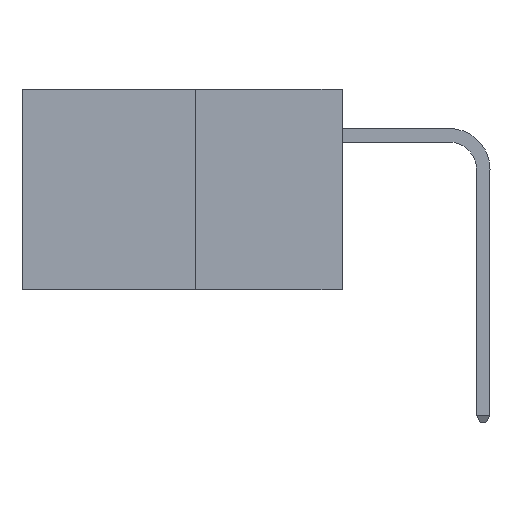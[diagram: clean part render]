
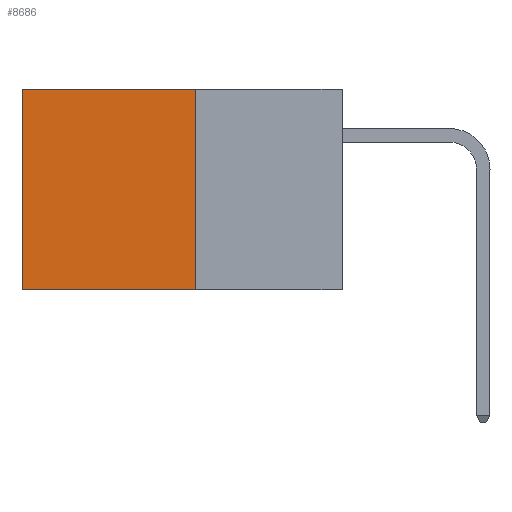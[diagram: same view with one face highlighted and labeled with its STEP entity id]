
A CAD part, left-side view. The second image highlights one B-rep face of the part: STEP entity #8686.
In plain terms, the highlighted planar face has unit normal (-1, 0, 0).
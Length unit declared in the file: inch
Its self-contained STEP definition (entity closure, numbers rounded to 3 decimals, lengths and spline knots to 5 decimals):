
#149 = LINE ( 'NONE', #12053, #574 ) ;
#518 = ORIENTED_EDGE ( 'NONE', *, *, #13031, .F. ) ;
#574 = VECTOR ( 'NONE', #11943, 39.37008 ) ;
#851 = CARTESIAN_POINT ( 'NONE',  ( 0.277, 0.27, 0. ) ) ;
#1091 = VERTEX_POINT ( 'NONE', #7757 ) ;
#2084 = VERTEX_POINT ( 'NONE', #6373 ) ;
#2275 = VERTEX_POINT ( 'NONE', #7153 ) ;
#2675 = DIRECTION ( 'NONE',  ( 1., 0., 0. ) ) ;
#2808 = LINE ( 'NONE', #12926, #16389 ) ;
#3205 = CARTESIAN_POINT ( 'NONE',  ( 0.277, 0.27, -0.37 ) ) ;
#3244 = VECTOR ( 'NONE', #12481, 39.37008 ) ;
#4827 = DIRECTION ( 'NONE',  ( 0., 1., 0. ) ) ;
#4994 = CARTESIAN_POINT ( 'NONE',  ( 0.277, 0.27, 0. ) ) ;
#5032 = EDGE_CURVE ( 'NONE', #2084, #2275, #149, .T. ) ;
#5058 = EDGE_CURVE ( 'NONE', #12966, #2084, #16876, .T. ) ;
#6373 = CARTESIAN_POINT ( 'NONE',  ( 0.277, 0.59, 0. ) ) ;
#6388 = LINE ( 'NONE', #3205, #3244 ) ;
#7064 = ORIENTED_EDGE ( 'NONE', *, *, #5058, .T. ) ;
#7153 = CARTESIAN_POINT ( 'NONE',  ( 0.277, 0.59, -0.37 ) ) ;
#7515 = ORIENTED_EDGE ( 'NONE', *, *, #13650, .F. ) ;
#7705 = DIRECTION ( 'NONE',  ( 0., 1., 0. ) ) ;
#7757 = CARTESIAN_POINT ( 'NONE',  ( 0.277, 0.27, -0.37 ) ) ;
#8004 = PLANE ( 'NONE',  #12241 ) ;
#8426 = ORIENTED_EDGE ( 'NONE', *, *, #5032, .T. ) ;
#8686 = ADVANCED_FACE ( 'NONE', ( #11304 ), #8004, .F. ) ;
#10797 = VECTOR ( 'NONE', #4827, 39.37008 ) ;
#11304 = FACE_OUTER_BOUND ( 'NONE', #13478, .T. ) ;
#11943 = DIRECTION ( 'NONE',  ( 0., 0., -1. ) ) ;
#11980 = DIRECTION ( 'NONE',  ( 0., 0., -1. ) ) ;
#12053 = CARTESIAN_POINT ( 'NONE',  ( 0.277, 0.59, -0.37 ) ) ;
#12241 = AXIS2_PLACEMENT_3D ( 'NONE', #17046, #2675, #11980 ) ;
#12481 = DIRECTION ( 'NONE',  ( 0., 0., -1. ) ) ;
#12926 = CARTESIAN_POINT ( 'NONE',  ( 0.277, 0.27, -0.37 ) ) ;
#12966 = VERTEX_POINT ( 'NONE', #851 ) ;
#13031 = EDGE_CURVE ( 'NONE', #1091, #2275, #2808, .T. ) ;
#13478 = EDGE_LOOP ( 'NONE', ( #8426, #518, #7515, #7064 ) ) ;
#13650 = EDGE_CURVE ( 'NONE', #12966, #1091, #6388, .T. ) ;
#16389 = VECTOR ( 'NONE', #7705, 39.37008 ) ;
#16876 = LINE ( 'NONE', #4994, #10797 ) ;
#17046 = CARTESIAN_POINT ( 'NONE',  ( 0.277, 0.27, -0.37 ) ) ;
